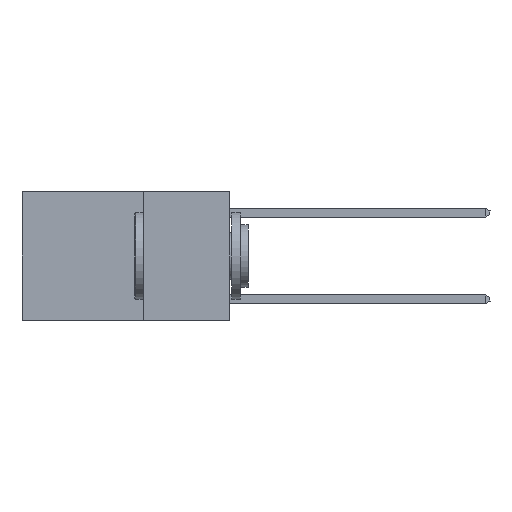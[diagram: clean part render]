
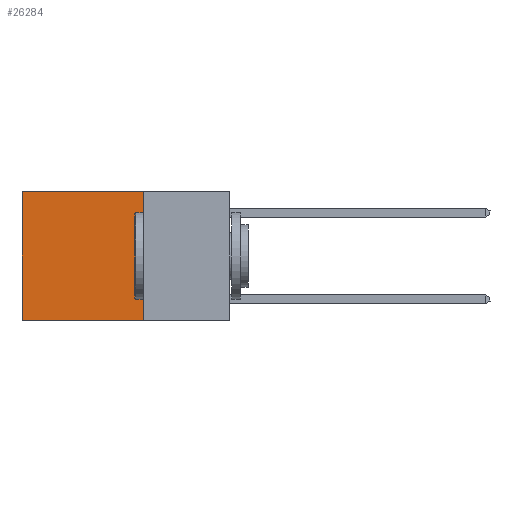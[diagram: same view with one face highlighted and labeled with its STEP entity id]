
A CAD part, left-side view. The second image highlights one B-rep face of the part: STEP entity #26284.
In plain terms, the highlighted planar face has unit normal (-1, 0, 0).
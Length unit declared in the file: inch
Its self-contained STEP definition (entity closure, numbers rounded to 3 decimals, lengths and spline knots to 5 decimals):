
#464 = DIRECTION ( 'NONE',  ( 0., 1., 0. ) ) ;
#1142 = CARTESIAN_POINT ( 'NONE',  ( 0.2625, 0.25, 0. ) ) ;
#2011 = EDGE_LOOP ( 'NONE', ( #17389, #23708, #13143, #22777 ) ) ;
#4192 = CARTESIAN_POINT ( 'NONE',  ( 0.2625, 0.25, 0. ) ) ;
#4590 = DIRECTION ( 'NONE',  ( 0., 0., -1. ) ) ;
#4724 = EDGE_CURVE ( 'NONE', #12355, #11944, #9452, .T. ) ;
#4861 = PLANE ( 'NONE',  #22863 ) ;
#7140 = FACE_OUTER_BOUND ( 'NONE', #2011, .T. ) ;
#8349 = VECTOR ( 'NONE', #13870, 39.37008 ) ;
#9019 = LINE ( 'NONE', #4192, #21481 ) ;
#9127 = LINE ( 'NONE', #9734, #12304 ) ;
#9452 = LINE ( 'NONE', #21188, #20082 ) ;
#9557 = CARTESIAN_POINT ( 'NONE',  ( 0.2625, 0.25, 0. ) ) ;
#9620 = CARTESIAN_POINT ( 'NONE',  ( 0.2625, 0.25, -0.37 ) ) ;
#9734 = CARTESIAN_POINT ( 'NONE',  ( 0.2625, 0.6, 0. ) ) ;
#11944 = VERTEX_POINT ( 'NONE', #21910 ) ;
#12304 = VECTOR ( 'NONE', #4590, 39.37008 ) ;
#12355 = VERTEX_POINT ( 'NONE', #1142 ) ;
#12585 = EDGE_CURVE ( 'NONE', #23171, #16775, #27761, .T. ) ;
#13143 = ORIENTED_EDGE ( 'NONE', *, *, #23024, .F. ) ;
#13153 = EDGE_CURVE ( 'NONE', #11944, #16775, #9127, .T. ) ;
#13870 = DIRECTION ( 'NONE',  ( 0., 1., 0. ) ) ;
#16775 = VERTEX_POINT ( 'NONE', #24845 ) ;
#17389 = ORIENTED_EDGE ( 'NONE', *, *, #13153, .T. ) ;
#18859 = DIRECTION ( 'NONE',  ( 1., 0., 0. ) ) ;
#20082 = VECTOR ( 'NONE', #464, 39.37008 ) ;
#20916 = DIRECTION ( 'NONE',  ( 0., 0., -1. ) ) ;
#21188 = CARTESIAN_POINT ( 'NONE',  ( 0.2625, 0.25, 0. ) ) ;
#21481 = VECTOR ( 'NONE', #20916, 39.37008 ) ;
#21910 = CARTESIAN_POINT ( 'NONE',  ( 0.2625, 0.6, 0. ) ) ;
#22777 = ORIENTED_EDGE ( 'NONE', *, *, #4724, .T. ) ;
#22863 = AXIS2_PLACEMENT_3D ( 'NONE', #9557, #18859, #28139 ) ;
#23024 = EDGE_CURVE ( 'NONE', #12355, #23171, #9019, .T. ) ;
#23171 = VERTEX_POINT ( 'NONE', #25769 ) ;
#23708 = ORIENTED_EDGE ( 'NONE', *, *, #12585, .F. ) ;
#24845 = CARTESIAN_POINT ( 'NONE',  ( 0.2625, 0.6, -0.37 ) ) ;
#25769 = CARTESIAN_POINT ( 'NONE',  ( 0.2625, 0.25, -0.37 ) ) ;
#26284 = ADVANCED_FACE ( 'NONE', ( #7140 ), #4861, .F. ) ;
#27761 = LINE ( 'NONE', #9620, #8349 ) ;
#28139 = DIRECTION ( 'NONE',  ( 0., 0., -1. ) ) ;
